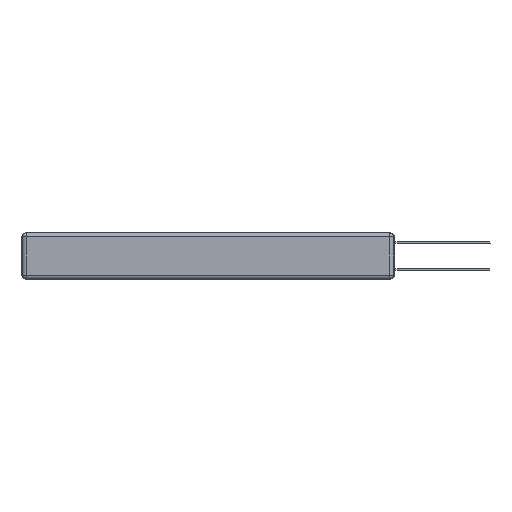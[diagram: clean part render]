
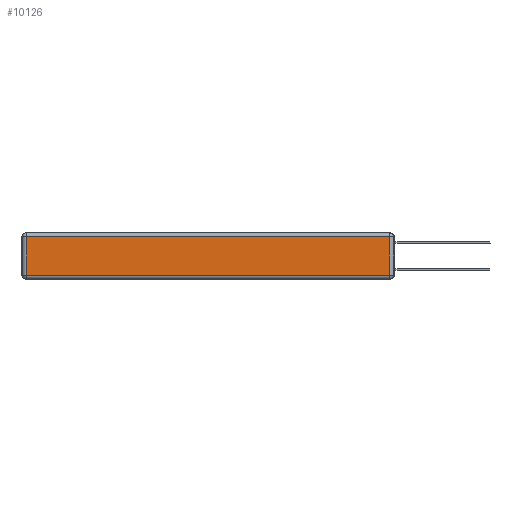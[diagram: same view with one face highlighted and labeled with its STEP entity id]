
A CAD part, left-side view. The second image highlights one B-rep face of the part: STEP entity #10126.
In plain terms, the highlighted planar face has unit normal (-1, 0, 0).
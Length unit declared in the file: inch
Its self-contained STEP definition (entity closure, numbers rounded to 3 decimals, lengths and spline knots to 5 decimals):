
#1703 = VERTEX_POINT ( 'NONE', #26984 ) ;
#1725 = EDGE_CURVE ( 'NONE', #2302, #3748, #10205, .T. ) ;
#2302 = VERTEX_POINT ( 'NONE', #20888 ) ;
#3748 = VERTEX_POINT ( 'NONE', #14919 ) ;
#4848 = EDGE_CURVE ( 'NONE', #15414, #1703, #10115, .T. ) ;
#5533 = DIRECTION ( 'NONE',  ( -1., 0., 0. ) ) ;
#5958 = DIRECTION ( 'NONE',  ( 0., 0., 1. ) ) ;
#6042 = ORIENTED_EDGE ( 'NONE', *, *, #17557, .T. ) ;
#7146 = EDGE_LOOP ( 'NONE', ( #17858, #24917, #6042, #11506 ) ) ;
#9416 = VECTOR ( 'NONE', #15095, 39.37008 ) ;
#10115 = LINE ( 'NONE', #18676, #23288 ) ;
#10126 = ADVANCED_FACE ( 'NONE', ( #10281 ), #19129, .T. ) ;
#10205 = LINE ( 'NONE', #21365, #15518 ) ;
#10281 = FACE_OUTER_BOUND ( 'NONE', #7146, .T. ) ;
#11506 = ORIENTED_EDGE ( 'NONE', *, *, #1725, .T. ) ;
#14919 = CARTESIAN_POINT ( 'NONE',  ( 0., 2.72, -0.313 ) ) ;
#15095 = DIRECTION ( 'NONE',  ( 0., 1., 0. ) ) ;
#15414 = VERTEX_POINT ( 'NONE', #20101 ) ;
#15518 = VECTOR ( 'NONE', #23234, 39.37008 ) ;
#17557 = EDGE_CURVE ( 'NONE', #1703, #2302, #26071, .T. ) ;
#17858 = ORIENTED_EDGE ( 'NONE', *, *, #22024, .T. ) ;
#18676 = CARTESIAN_POINT ( 'NONE',  ( 0., 0.03, -0.343 ) ) ;
#19129 = PLANE ( 'NONE',  #22077 ) ;
#19870 = CARTESIAN_POINT ( 'NONE',  ( 0., 0., -0.313 ) ) ;
#20006 = VECTOR ( 'NONE', #22311, 39.37008 ) ;
#20101 = CARTESIAN_POINT ( 'NONE',  ( 0., 0.03, -0.313 ) ) ;
#20158 = LINE ( 'NONE', #19870, #20006 ) ;
#20888 = CARTESIAN_POINT ( 'NONE',  ( 0., 2.72, -0.03 ) ) ;
#21365 = CARTESIAN_POINT ( 'NONE',  ( 0., 2.72, -0.343 ) ) ;
#22024 = EDGE_CURVE ( 'NONE', #3748, #15414, #20158, .T. ) ;
#22077 = AXIS2_PLACEMENT_3D ( 'NONE', #27924, #5533, #5958 ) ;
#22311 = DIRECTION ( 'NONE',  ( 0., -1., 0. ) ) ;
#23234 = DIRECTION ( 'NONE',  ( 0., 0., -1. ) ) ;
#23288 = VECTOR ( 'NONE', #25168, 39.37008 ) ;
#24917 = ORIENTED_EDGE ( 'NONE', *, *, #4848, .T. ) ;
#25168 = DIRECTION ( 'NONE',  ( 0., 0., 1. ) ) ;
#26071 = LINE ( 'NONE', #26209, #9416 ) ;
#26209 = CARTESIAN_POINT ( 'NONE',  ( 0., 2.75, -0.03 ) ) ;
#26984 = CARTESIAN_POINT ( 'NONE',  ( 0., 0.03, -0.03 ) ) ;
#27924 = CARTESIAN_POINT ( 'NONE',  ( 0., 0., -0.343 ) ) ;
